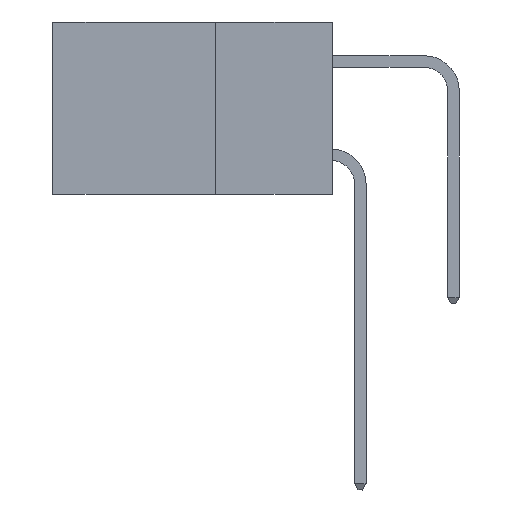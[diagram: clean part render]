
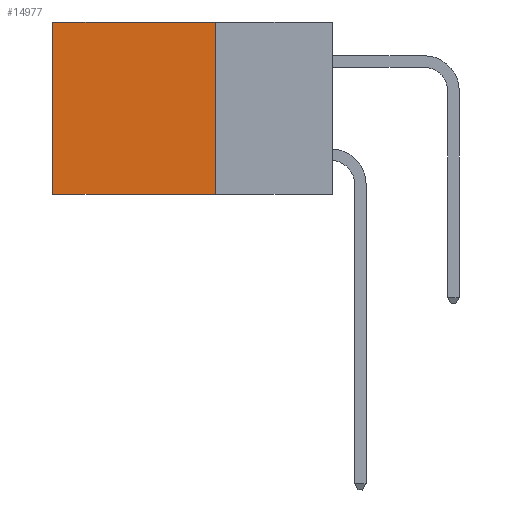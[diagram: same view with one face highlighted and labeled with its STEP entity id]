
A CAD part, left-side view. The second image highlights one B-rep face of the part: STEP entity #14977.
In plain terms, the highlighted planar face has unit normal (-1, 0, 0).
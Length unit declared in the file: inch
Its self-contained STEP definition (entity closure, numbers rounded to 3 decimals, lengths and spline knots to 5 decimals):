
#63 = CARTESIAN_POINT ( 'NONE',  ( 0.298, 0.25, -0.37 ) ) ;
#666 = DIRECTION ( 'NONE',  ( 0., 0., -1. ) ) ;
#1377 = LINE ( 'NONE', #11949, #15259 ) ;
#1656 = VERTEX_POINT ( 'NONE', #15556 ) ;
#1867 = ORIENTED_EDGE ( 'NONE', *, *, #6258, .T. ) ;
#2253 = ORIENTED_EDGE ( 'NONE', *, *, #19055, .F. ) ;
#2340 = CARTESIAN_POINT ( 'NONE',  ( 0.298, 0.25, 0. ) ) ;
#2386 = DIRECTION ( 'NONE',  ( 0., 1., 0. ) ) ;
#2525 = CARTESIAN_POINT ( 'NONE',  ( 0.298, 0.6, 0. ) ) ;
#2724 = VERTEX_POINT ( 'NONE', #12116 ) ;
#6258 = EDGE_CURVE ( 'NONE', #2724, #13319, #1377, .T. ) ;
#7879 = CARTESIAN_POINT ( 'NONE',  ( 0.298, 0.6, 0. ) ) ;
#9779 = DIRECTION ( 'NONE',  ( 0., 0., -1. ) ) ;
#10015 = DIRECTION ( 'NONE',  ( 0., 1., 0. ) ) ;
#10559 = VECTOR ( 'NONE', #666, 39.37008 ) ;
#10960 = EDGE_CURVE ( 'NONE', #13319, #1656, #20730, .T. ) ;
#11949 = CARTESIAN_POINT ( 'NONE',  ( 0.298, 0.25, 0. ) ) ;
#12116 = CARTESIAN_POINT ( 'NONE',  ( 0.298, 0.25, 0. ) ) ;
#12342 = CARTESIAN_POINT ( 'NONE',  ( 0.298, 0.25, -0.37 ) ) ;
#12974 = VECTOR ( 'NONE', #15939, 39.37008 ) ;
#13002 = PLANE ( 'NONE',  #18513 ) ;
#13319 = VERTEX_POINT ( 'NONE', #2525 ) ;
#13931 = EDGE_LOOP ( 'NONE', ( #16798, #2253, #14525, #1867 ) ) ;
#14525 = ORIENTED_EDGE ( 'NONE', *, *, #21063, .F. ) ;
#14668 = DIRECTION ( 'NONE',  ( 1., 0., 0. ) ) ;
#14977 = ADVANCED_FACE ( 'NONE', ( #19877 ), #13002, .F. ) ;
#15259 = VECTOR ( 'NONE', #2386, 39.37008 ) ;
#15494 = LINE ( 'NONE', #63, #18838 ) ;
#15556 = CARTESIAN_POINT ( 'NONE',  ( 0.298, 0.6, -0.37 ) ) ;
#15939 = DIRECTION ( 'NONE',  ( 0., 0., -1. ) ) ;
#16798 = ORIENTED_EDGE ( 'NONE', *, *, #10960, .T. ) ;
#17859 = CARTESIAN_POINT ( 'NONE',  ( 0.298, 0.25, 0. ) ) ;
#18032 = LINE ( 'NONE', #2340, #10559 ) ;
#18513 = AXIS2_PLACEMENT_3D ( 'NONE', #17859, #14668, #9779 ) ;
#18838 = VECTOR ( 'NONE', #10015, 39.37008 ) ;
#19055 = EDGE_CURVE ( 'NONE', #20588, #1656, #15494, .T. ) ;
#19877 = FACE_OUTER_BOUND ( 'NONE', #13931, .T. ) ;
#20588 = VERTEX_POINT ( 'NONE', #12342 ) ;
#20730 = LINE ( 'NONE', #7879, #12974 ) ;
#21063 = EDGE_CURVE ( 'NONE', #2724, #20588, #18032, .T. ) ;
